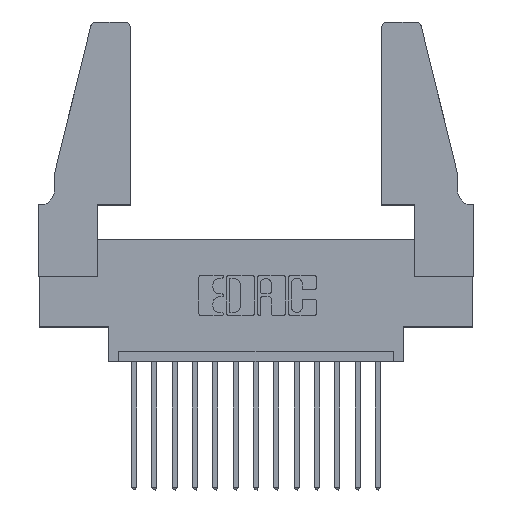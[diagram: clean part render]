
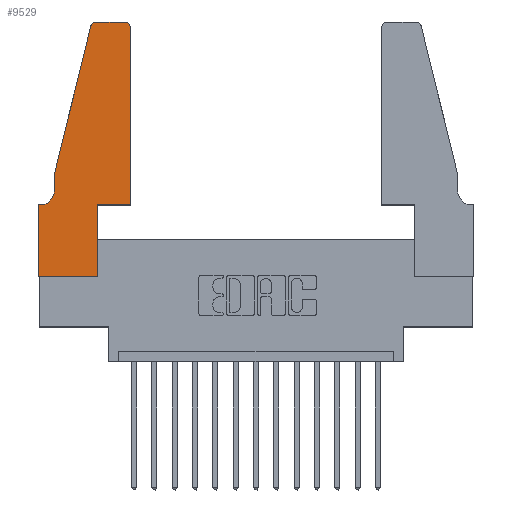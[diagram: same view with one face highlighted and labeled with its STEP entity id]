
A CAD part, top view. The second image highlights one B-rep face of the part: STEP entity #9529.
In plain terms, the highlighted planar face has unit normal (0, 0, 1).
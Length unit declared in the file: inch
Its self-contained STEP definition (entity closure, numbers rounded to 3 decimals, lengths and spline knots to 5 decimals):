
#797 = DIRECTION ( 'NONE',  ( 1., 0., 0. ) ) ;
#810 = EDGE_CURVE ( 'NONE', #11974, #15993, #15308, .T. ) ;
#885 = VERTEX_POINT ( 'NONE', #5635 ) ;
#930 = CARTESIAN_POINT ( 'NONE',  ( 0.2865, 0., 0.37 ) ) ;
#1323 = ORIENTED_EDGE ( 'NONE', *, *, #15444, .T. ) ;
#1387 = DIRECTION ( 'NONE',  ( -1., 0., 0. ) ) ;
#1624 = VERTEX_POINT ( 'NONE', #10596 ) ;
#1670 = PLANE ( 'NONE',  #6991 ) ;
#1701 = VERTEX_POINT ( 'NONE', #5760 ) ;
#1799 = EDGE_CURVE ( 'NONE', #1701, #12964, #9984, .T. ) ;
#2120 = CIRCLE ( 'NONE', #10947, 0.03 ) ;
#2623 = FACE_OUTER_BOUND ( 'NONE', #13615, .T. ) ;
#3022 = EDGE_CURVE ( 'NONE', #12964, #11142, #14174, .T. ) ;
#3226 = CARTESIAN_POINT ( 'NONE',  ( 0.284, 1.22, 0.37 ) ) ;
#3805 = AXIS2_PLACEMENT_3D ( 'NONE', #3226, #8211, #797 ) ;
#4052 = ORIENTED_EDGE ( 'NONE', *, *, #6835, .T. ) ;
#4106 = CARTESIAN_POINT ( 'NONE',  ( 0., 0.35, 0.37 ) ) ;
#4159 = VECTOR ( 'NONE', #8589, 39.37008 ) ;
#4176 = CARTESIAN_POINT ( 'NONE',  ( 0.2865, 0.35, 0.37 ) ) ;
#4251 = CARTESIAN_POINT ( 'NONE',  ( 0., 0., 0.37 ) ) ;
#4326 = CARTESIAN_POINT ( 'NONE',  ( 0.0755, 0.5, 0.37 ) ) ;
#4944 = EDGE_CURVE ( 'NONE', #15993, #9242, #9455, .T. ) ;
#4988 = VERTEX_POINT ( 'NONE', #5946 ) ;
#5273 = ORIENTED_EDGE ( 'NONE', *, *, #1799, .T. ) ;
#5306 = DIRECTION ( 'NONE',  ( 0., 0., 1. ) ) ;
#5635 = CARTESIAN_POINT ( 'NONE',  ( 0.0755, 0.5, 0.37 ) ) ;
#5659 = EDGE_CURVE ( 'NONE', #4988, #11514, #9077, .T. ) ;
#5760 = CARTESIAN_POINT ( 'NONE',  ( 0.4205, 1.25, 0.37 ) ) ;
#5946 = CARTESIAN_POINT ( 'NONE',  ( 0., 0.35, 0.37 ) ) ;
#6063 = LINE ( 'NONE', #15338, #6663 ) ;
#6301 = EDGE_CURVE ( 'NONE', #11142, #885, #9804, .T. ) ;
#6375 = CARTESIAN_POINT ( 'NONE',  ( 0.284, 1.25, 0.37 ) ) ;
#6526 = DIRECTION ( 'NONE',  ( 0., -1., 0. ) ) ;
#6602 = LINE ( 'NONE', #4251, #14507 ) ;
#6639 = CARTESIAN_POINT ( 'NONE',  ( 0.2865, 0.35, 0.37 ) ) ;
#6663 = VECTOR ( 'NONE', #12959, 39.37008 ) ;
#6685 = LINE ( 'NONE', #15964, #4159 ) ;
#6835 = EDGE_CURVE ( 'NONE', #885, #11952, #6685, .T. ) ;
#6991 = AXIS2_PLACEMENT_3D ( 'NONE', #4106, #5306, #9170 ) ;
#7185 = AXIS2_PLACEMENT_3D ( 'NONE', #12601, #14854, #1387 ) ;
#7299 = EDGE_CURVE ( 'NONE', #11514, #11974, #6602, .T. ) ;
#7317 = DIRECTION ( 'NONE',  ( -1., 0., 0. ) ) ;
#7351 = DIRECTION ( 'NONE',  ( -1., 0., 0. ) ) ;
#8032 = VECTOR ( 'NONE', #7351, 39.37008 ) ;
#8211 = DIRECTION ( 'NONE',  ( 0., 0., 1. ) ) ;
#8589 = DIRECTION ( 'NONE',  ( 0., -1., 0. ) ) ;
#8774 = CARTESIAN_POINT ( 'NONE',  ( 0.0755, 0.35, 0.37 ) ) ;
#8783 = VERTEX_POINT ( 'NONE', #11296 ) ;
#9077 = LINE ( 'NONE', #12586, #15239 ) ;
#9091 = VECTOR ( 'NONE', #11981, 39.37008 ) ;
#9170 = DIRECTION ( 'NONE',  ( 1., 0., 0. ) ) ;
#9216 = DIRECTION ( 'NONE',  ( 1., 0., 0. ) ) ;
#9242 = VERTEX_POINT ( 'NONE', #12186 ) ;
#9356 = DIRECTION ( 'NONE',  ( 1., 0., 0. ) ) ;
#9455 = LINE ( 'NONE', #13251, #9091 ) ;
#9529 = ADVANCED_FACE ( 'NONE', ( #2623 ), #1670, .T. ) ;
#9579 = LINE ( 'NONE', #8774, #8032 ) ;
#9791 = EDGE_CURVE ( 'NONE', #1624, #4988, #9579, .T. ) ;
#9804 = LINE ( 'NONE', #4326, #14242 ) ;
#9839 = CARTESIAN_POINT ( 'NONE',  ( 0., 0., 0.37 ) ) ;
#9984 = LINE ( 'NONE', #14706, #10738 ) ;
#10284 = ORIENTED_EDGE ( 'NONE', *, *, #810, .T. ) ;
#10447 = ORIENTED_EDGE ( 'NONE', *, *, #4944, .T. ) ;
#10544 = CIRCLE ( 'NONE', #7185, 0.07 ) ;
#10555 = CARTESIAN_POINT ( 'NONE',  ( 0.4205, 1.22, 0.37 ) ) ;
#10596 = CARTESIAN_POINT ( 'NONE',  ( 0.0055, 0.35, 0.37 ) ) ;
#10738 = VECTOR ( 'NONE', #7317, 39.37008 ) ;
#10792 = CARTESIAN_POINT ( 'NONE',  ( 0.0755, 0.42, 0.37 ) ) ;
#10947 = AXIS2_PLACEMENT_3D ( 'NONE', #10555, #14320, #9216 ) ;
#11089 = EDGE_CURVE ( 'NONE', #11952, #1624, #10544, .T. ) ;
#11142 = VERTEX_POINT ( 'NONE', #12656 ) ;
#11296 = CARTESIAN_POINT ( 'NONE',  ( 0.4505, 1.22, 0.37 ) ) ;
#11514 = VERTEX_POINT ( 'NONE', #9839 ) ;
#11574 = ORIENTED_EDGE ( 'NONE', *, *, #3022, .T. ) ;
#11952 = VERTEX_POINT ( 'NONE', #10792 ) ;
#11974 = VERTEX_POINT ( 'NONE', #930 ) ;
#11981 = DIRECTION ( 'NONE',  ( 1., 0., 0. ) ) ;
#12186 = CARTESIAN_POINT ( 'NONE',  ( 0.4505, 0.35, 0.37 ) ) ;
#12586 = CARTESIAN_POINT ( 'NONE',  ( 0., 0., 0.37 ) ) ;
#12601 = CARTESIAN_POINT ( 'NONE',  ( 0.0055, 0.42, 0.37 ) ) ;
#12656 = CARTESIAN_POINT ( 'NONE',  ( 0.25487, 1.22718, 0.37 ) ) ;
#12785 = DIRECTION ( 'NONE',  ( 0., 1., 0. ) ) ;
#12959 = DIRECTION ( 'NONE',  ( 0., 1., 0. ) ) ;
#12964 = VERTEX_POINT ( 'NONE', #6375 ) ;
#12967 = ORIENTED_EDGE ( 'NONE', *, *, #7299, .T. ) ;
#12980 = VECTOR ( 'NONE', #12785, 39.37008 ) ;
#12998 = DIRECTION ( 'NONE',  ( -0.239, -0.971, 0. ) ) ;
#13127 = ORIENTED_EDGE ( 'NONE', *, *, #5659, .T. ) ;
#13251 = CARTESIAN_POINT ( 'NONE',  ( 0.4505, 0.35, 0.37 ) ) ;
#13522 = ORIENTED_EDGE ( 'NONE', *, *, #11089, .T. ) ;
#13615 = EDGE_LOOP ( 'NONE', ( #5273, #11574, #15920, #4052, #13522, #13754, #13127, #12967, #10284, #10447, #13660, #1323 ) ) ;
#13660 = ORIENTED_EDGE ( 'NONE', *, *, #14308, .T. ) ;
#13754 = ORIENTED_EDGE ( 'NONE', *, *, #9791, .T. ) ;
#14174 = CIRCLE ( 'NONE', #3805, 0.03 ) ;
#14242 = VECTOR ( 'NONE', #12998, 39.37008 ) ;
#14308 = EDGE_CURVE ( 'NONE', #9242, #8783, #6063, .T. ) ;
#14320 = DIRECTION ( 'NONE',  ( 0., 0., 1. ) ) ;
#14507 = VECTOR ( 'NONE', #9356, 39.37008 ) ;
#14706 = CARTESIAN_POINT ( 'NONE',  ( 0.2605, 1.25, 0.37 ) ) ;
#14854 = DIRECTION ( 'NONE',  ( 0., 0., -1. ) ) ;
#15239 = VECTOR ( 'NONE', #6526, 39.37008 ) ;
#15308 = LINE ( 'NONE', #4176, #12980 ) ;
#15338 = CARTESIAN_POINT ( 'NONE',  ( 0.4505, 0.35, 0.37 ) ) ;
#15444 = EDGE_CURVE ( 'NONE', #8783, #1701, #2120, .T. ) ;
#15920 = ORIENTED_EDGE ( 'NONE', *, *, #6301, .T. ) ;
#15964 = CARTESIAN_POINT ( 'NONE',  ( 0.0755, 0.5, 0.37 ) ) ;
#15993 = VERTEX_POINT ( 'NONE', #6639 ) ;
